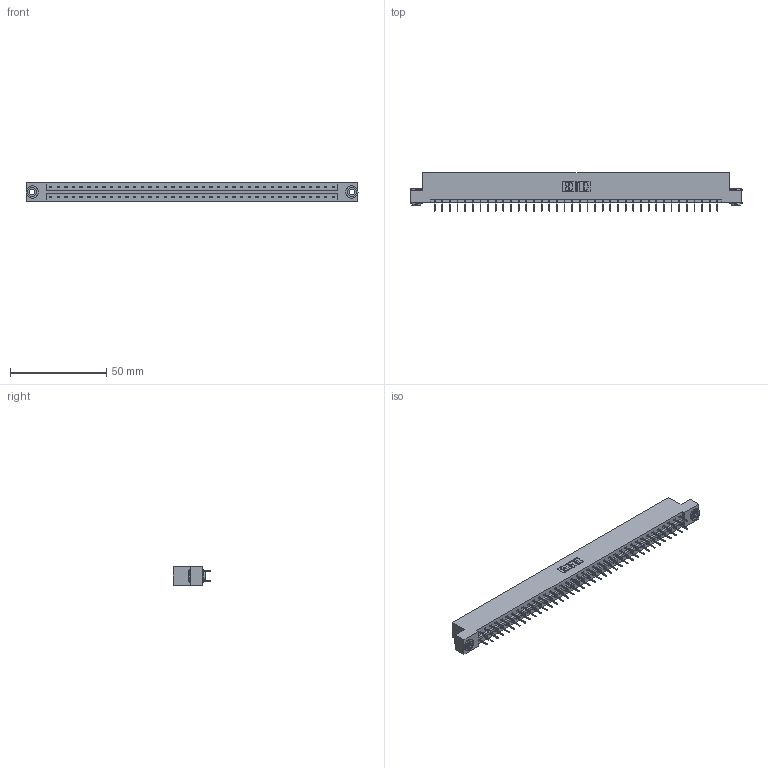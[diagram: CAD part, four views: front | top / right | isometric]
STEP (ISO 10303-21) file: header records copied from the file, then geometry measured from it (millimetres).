
FILE_DESCRIPTION (( 'STEP AP203' ), '1' );
FILE_NAME ('833-076-524-203.STEP', '2020-06-05T18:10:15', ( '' ), ( '' ), 'SwSTEP 2.0', 'SolidWorks 2020', '' );
FILE_SCHEMA (( 'CONFIG_CONTROL_DESIGN' ));
Length unit declared in the file: inch
Products named in the file (4): 833-076-524-203; 345-250-002_345-250-002-102; 833 Part_Flush - .156 Dia - TH; 345-292-001_345-293-124
Assembly tree (79 placements, depth 2):
  833-076-524-203
    833 Part_Flush - .156 Dia - TH
    345-292-001_345-293-124  x76
    345-250-002_345-250-002-102  x2
Bounding box: 172.11 x 19.69 x 9.4 mm (x, y, z)
Volume: 17438.5 mm3; surface area: 20449.3 mm2
Topology: 79 solids, 79 shells, 4408 faces, 12471 edges, 8006 vertices
Faces by surface type: plane 3272, cylinder 1128, cone 8
Entity records: 25688 total; most frequent: CARTESIAN_POINT 4237, ORIENTED_EDGE 4166, DIRECTION 3661, EDGE_CURVE 2083, VECTOR 1935, LINE 1935, VERTEX_POINT 1382, AXIS2_PLACEMENT_3D 863
